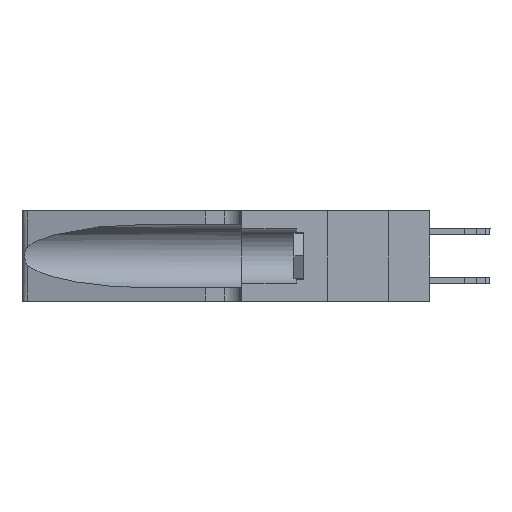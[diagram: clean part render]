
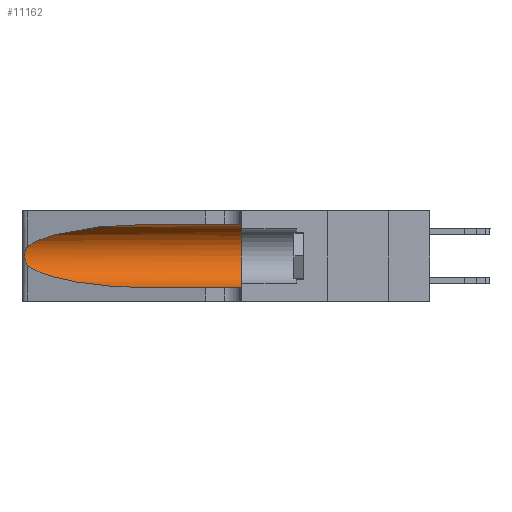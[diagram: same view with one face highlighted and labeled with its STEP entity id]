
A CAD part, left-side view. The second image highlights one B-rep face of the part: STEP entity #11162.
In plain terms, the highlighted cylindrical face has radius 3.308 mm (diameter 6.617 mm), a partial arc.
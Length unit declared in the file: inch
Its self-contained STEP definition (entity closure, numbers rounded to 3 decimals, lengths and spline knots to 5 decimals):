
#324 = CARTESIAN_POINT ( 'NONE',  ( 0.18966, 0.96281, 0.31525 ) ) ;
#360 = EDGE_LOOP ( 'NONE', ( #4001, #486, #7696, #11745, #9903, #6083 ) ) ;
#420 = VERTEX_POINT ( 'NONE', #11914 ) ;
#486 = ORIENTED_EDGE ( 'NONE', *, *, #1289, .T. ) ;
#699 = EDGE_CURVE ( 'NONE', #8073, #9259, #14118, .T. ) ;
#720 = CYLINDRICAL_SURFACE ( 'NONE', #15241, 0.13025 ) ;
#892 = CARTESIAN_POINT ( 'NONE',  ( 0.25487, 1.22718, 0.14631 ) ) ;
#1170 = AXIS2_PLACEMENT_3D ( 'NONE', #5191, #14178, #17093 ) ;
#1289 = EDGE_CURVE ( 'NONE', #9259, #420, #17041, .T. ) ;
#1757 = VERTEX_POINT ( 'NONE', #7133 ) ;
#2342 = CARTESIAN_POINT ( 'NONE',  ( 0.2373, 1.15595, 0.08982 ) ) ;
#2419 = DIRECTION ( 'NONE',  ( 0., 0., -1. ) ) ;
#3146 = CARTESIAN_POINT ( 'NONE',  ( 0.25487, 1.22718, 0.14631 ) ) ;
#4001 = ORIENTED_EDGE ( 'NONE', *, *, #699, .T. ) ;
#4283 = EDGE_CURVE ( 'NONE', #420, #16726, #17656, .T. ) ;
#4598 = CARTESIAN_POINT ( 'NONE',  ( 0.25789, 1.23486, 0.15765 ) ) ;
#4727 = CARTESIAN_POINT ( 'NONE',  ( 0.25639, 1.23186, 0.15144 ) ) ;
#5191 = CARTESIAN_POINT ( 'NONE',  ( 0.1305, 0.35, 0.185 ) ) ;
#6083 = ORIENTED_EDGE ( 'NONE', *, *, #9421, .F. ) ;
#6198 = CARTESIAN_POINT ( 'NONE',  ( 0.25555, 1.22994, 0.2215 ) ) ;
#6334 = CARTESIAN_POINT ( 'NONE',  ( 0.26018, 1.23835, 0.19895 ) ) ;
#7133 = CARTESIAN_POINT ( 'NONE',  ( 0.1305, 0.35, 0.31525 ) ) ;
#7673 = CARTESIAN_POINT ( 'NONE',  ( 0.25787, 1.23484, 0.2124 ) ) ;
#7696 = ORIENTED_EDGE ( 'NONE', *, *, #4283, .T. ) ;
#7938 = CARTESIAN_POINT ( 'NONE',  ( 0.25487, 1.22718, 0.22369 ) ) ;
#8073 = VERTEX_POINT ( 'NONE', #15541 ) ;
#8393 = CARTESIAN_POINT ( 'NONE',  ( 0.18966, 0.96281, 0.05475 ) ) ;
#8549 = DIRECTION ( 'NONE',  ( 0., -1., 0. ) ) ;
#9259 = VERTEX_POINT ( 'NONE', #7938 ) ;
#9421 = EDGE_CURVE ( 'NONE', #8073, #1757, #10477, .T. ) ;
#9903 = ORIENTED_EDGE ( 'NONE', *, *, #17735, .F. ) ;
#9911 = CARTESIAN_POINT ( 'NONE',  ( 0.1305, 1.61858, 0.185 ) ) ;
#10477 = LINE ( 'NONE', #12883, #12134 ) ;
#10673 = FACE_OUTER_BOUND ( 'NONE', #360, .T. ) ;
#10699 = CARTESIAN_POINT ( 'NONE',  ( 0.25639, 1.23184, 0.21858 ) ) ;
#10767 = CARTESIAN_POINT ( 'NONE',  ( 0.25854, 1.2359, 0.20912 ) ) ;
#10888 = CARTESIAN_POINT ( 'NONE',  ( 0.25856, 1.23593, 0.16098 ) ) ;
#10915 = LINE ( 'NONE', #14675, #11390 ) ;
#10973 = CARTESIAN_POINT ( 'NONE',  ( 0.1305, 0.72297, 0.31525 ) ) ;
#11162 = ADVANCED_FACE ( 'NONE', ( #10673 ), #720, .F. ) ;
#11390 = VECTOR ( 'NONE', #11514, 39.37008 ) ;
#11469 = CARTESIAN_POINT ( 'NONE',  ( 0.1305, 0.72297, 0.05475 ) ) ;
#11514 = DIRECTION ( 'NONE',  ( 0., -1., 0. ) ) ;
#11745 = ORIENTED_EDGE ( 'NONE', *, *, #17269, .T. ) ;
#11914 = CARTESIAN_POINT ( 'NONE',  ( 0.25487, 1.22718, 0.14631 ) ) ;
#12134 = VECTOR ( 'NONE', #8549, 39.37008 ) ;
#12279 = CARTESIAN_POINT ( 'NONE',  ( 0.26075, 1.23896, 0.178 ) ) ;
#12396 = CARTESIAN_POINT ( 'NONE',  ( 0.26017, 1.23833, 0.17102 ) ) ;
#12791 = CIRCLE ( 'NONE', #1170, 0.13025 ) ;
#12883 = CARTESIAN_POINT ( 'NONE',  ( 0.1305, 1.61858, 0.31525 ) ) ;
#13725 = CARTESIAN_POINT ( 'NONE',  ( 0.25487, 1.22718, 0.22369 ) ) ;
#13858 = CARTESIAN_POINT ( 'NONE',  ( 0.25555, 1.22993, 0.14849 ) ) ;
#14118 =( BOUNDED_CURVE ( )  B_SPLINE_CURVE ( 3, ( #10973, #324, #14133, #15379 ),
 .UNSPECIFIED., .F., .F. ) 
 B_SPLINE_CURVE_WITH_KNOTS ( ( 4, 4 ),
 ( 1.5708, 2.84003 ),
 .UNSPECIFIED. ) 
 CURVE ( )  GEOMETRIC_REPRESENTATION_ITEM ( )  RATIONAL_B_SPLINE_CURVE ( ( 1., 0.87, 0.87, 1. ) ) 
 REPRESENTATION_ITEM ( '' )  );
#14133 = CARTESIAN_POINT ( 'NONE',  ( 0.2373, 1.15595, 0.28018 ) ) ;
#14178 = DIRECTION ( 'NONE',  ( 0., 1., 0. ) ) ;
#14675 = CARTESIAN_POINT ( 'NONE',  ( 0.1305, 1.61858, 0.05475 ) ) ;
#15241 = AXIS2_PLACEMENT_3D ( 'NONE', #9911, #18997, #2419 ) ;
#15379 = CARTESIAN_POINT ( 'NONE',  ( 0.25487, 1.22718, 0.22369 ) ) ;
#15541 = CARTESIAN_POINT ( 'NONE',  ( 0.1305, 0.72297, 0.31525 ) ) ;
#15800 = CARTESIAN_POINT ( 'NONE',  ( 0.1305, 0.35, 0.05475 ) ) ;
#16492 = CARTESIAN_POINT ( 'NONE',  ( 0.1305, 0.72297, 0.05475 ) ) ;
#16726 = VERTEX_POINT ( 'NONE', #16492 ) ;
#16766 = CARTESIAN_POINT ( 'NONE',  ( 0.26075, 1.23896, 0.19203 ) ) ;
#17041 = B_SPLINE_CURVE_WITH_KNOTS ( 'NONE', 3,
 ( #13725, #6198, #10699, #7673, #10767, #6334, #16766, #12279, #12396, #10888, #4598, #4727, #13858, #3146 ),
 .UNSPECIFIED., .F., .F.,
 ( 4, 2, 2, 2, 2, 2, 4 ),
 ( 0., 0.00027, 0.00053, 0.00107, 0.0016, 0.00187, 0.00214 ),
 .UNSPECIFIED. ) ;
#17093 = DIRECTION ( 'NONE',  ( 0., 0., 1. ) ) ;
#17239 = VERTEX_POINT ( 'NONE', #15800 ) ;
#17269 = EDGE_CURVE ( 'NONE', #16726, #17239, #10915, .T. ) ;
#17656 =( BOUNDED_CURVE ( )  B_SPLINE_CURVE ( 3, ( #892, #2342, #8393, #11469 ),
 .UNSPECIFIED., .F., .T. ) 
 B_SPLINE_CURVE_WITH_KNOTS ( ( 4, 4 ),
 ( 3.44316, 4.71239 ),
 .UNSPECIFIED. ) 
 CURVE ( )  GEOMETRIC_REPRESENTATION_ITEM ( )  RATIONAL_B_SPLINE_CURVE ( ( 1., 0.87, 0.87, 1. ) ) 
 REPRESENTATION_ITEM ( '' )  );
#17735 = EDGE_CURVE ( 'NONE', #1757, #17239, #12791, .T. ) ;
#18997 = DIRECTION ( 'NONE',  ( 0., -1., 0. ) ) ;
